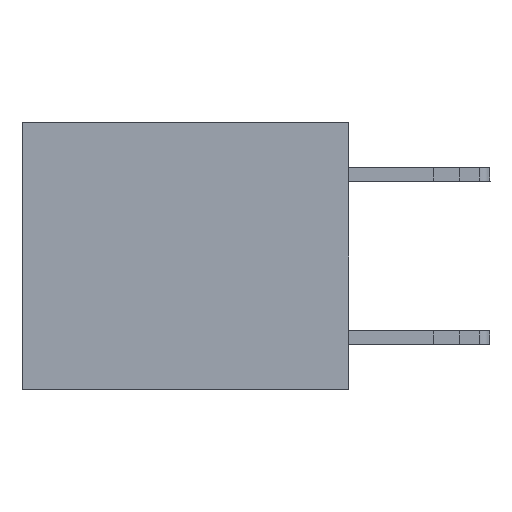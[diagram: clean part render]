
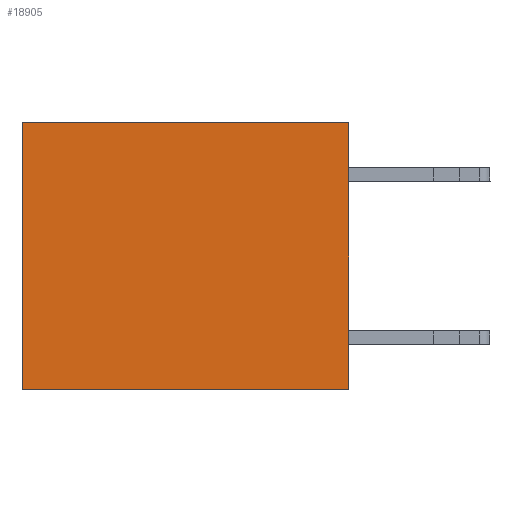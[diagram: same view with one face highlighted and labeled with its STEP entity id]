
A CAD part, left-side view. The second image highlights one B-rep face of the part: STEP entity #18905.
In plain terms, the highlighted planar face has unit normal (-1, 0, 0).
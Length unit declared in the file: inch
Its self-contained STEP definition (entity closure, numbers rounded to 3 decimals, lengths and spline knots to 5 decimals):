
#299 = EDGE_CURVE ( 'NONE', #15419, #5548, #28217, .T. ) ;
#570 = CARTESIAN_POINT ( 'NONE',  ( 0.3165, 0., -0.49 ) ) ;
#3374 = DIRECTION ( 'NONE',  ( 0., 0., -1. ) ) ;
#4100 = DIRECTION ( 'NONE',  ( 0., 1., 0. ) ) ;
#5244 = CARTESIAN_POINT ( 'NONE',  ( 0.3165, 0., -0.49 ) ) ;
#5548 = VERTEX_POINT ( 'NONE', #22096 ) ;
#7790 = EDGE_CURVE ( 'NONE', #15396, #23999, #29024, .T. ) ;
#9704 = DIRECTION ( 'NONE',  ( 1., 0., 0. ) ) ;
#9738 = CARTESIAN_POINT ( 'NONE',  ( 0.3165, 0., -0.49 ) ) ;
#10793 = CARTESIAN_POINT ( 'NONE',  ( 0.3165, 0., 0. ) ) ;
#13376 = CARTESIAN_POINT ( 'NONE',  ( 0.3165, 0.6, -0.49 ) ) ;
#13514 = CARTESIAN_POINT ( 'NONE',  ( 0.3165, 0.6, -0.49 ) ) ;
#15396 = VERTEX_POINT ( 'NONE', #570 ) ;
#15419 = VERTEX_POINT ( 'NONE', #15580 ) ;
#15580 = CARTESIAN_POINT ( 'NONE',  ( 0.3165, 0., 0. ) ) ;
#15620 = VECTOR ( 'NONE', #3374, 39.37008 ) ;
#16454 = VECTOR ( 'NONE', #4100, 39.37008 ) ;
#17213 = DIRECTION ( 'NONE',  ( 0., 0., -1. ) ) ;
#17348 = DIRECTION ( 'NONE',  ( 0., 0., -1. ) ) ;
#17534 = PLANE ( 'NONE',  #19337 ) ;
#17931 = EDGE_LOOP ( 'NONE', ( #21598, #27210, #29148, #20636 ) ) ;
#18905 = ADVANCED_FACE ( 'NONE', ( #21263 ), #17534, .F. ) ;
#19177 = VECTOR ( 'NONE', #17348, 39.37008 ) ;
#19337 = AXIS2_PLACEMENT_3D ( 'NONE', #5244, #9704, #17213 ) ;
#20636 = ORIENTED_EDGE ( 'NONE', *, *, #299, .T. ) ;
#21263 = FACE_OUTER_BOUND ( 'NONE', #17931, .T. ) ;
#21495 = VECTOR ( 'NONE', #28320, 39.37008 ) ;
#21598 = ORIENTED_EDGE ( 'NONE', *, *, #24504, .T. ) ;
#22096 = CARTESIAN_POINT ( 'NONE',  ( 0.3165, 0.6, 0. ) ) ;
#23647 = EDGE_CURVE ( 'NONE', #15419, #15396, #27844, .T. ) ;
#23822 = LINE ( 'NONE', #13376, #15620 ) ;
#23999 = VERTEX_POINT ( 'NONE', #13514 ) ;
#24504 = EDGE_CURVE ( 'NONE', #5548, #23999, #23822, .T. ) ;
#27210 = ORIENTED_EDGE ( 'NONE', *, *, #7790, .F. ) ;
#27844 = LINE ( 'NONE', #9738, #19177 ) ;
#28217 = LINE ( 'NONE', #10793, #21495 ) ;
#28320 = DIRECTION ( 'NONE',  ( 0., 1., 0. ) ) ;
#29024 = LINE ( 'NONE', #32277, #16454 ) ;
#29148 = ORIENTED_EDGE ( 'NONE', *, *, #23647, .F. ) ;
#32277 = CARTESIAN_POINT ( 'NONE',  ( 0.3165, 0., -0.49 ) ) ;
